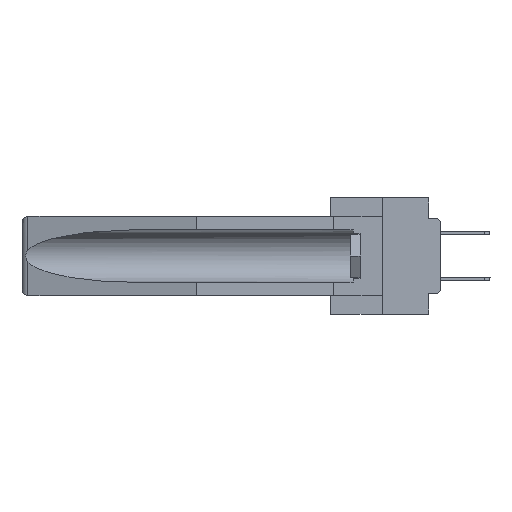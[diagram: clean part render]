
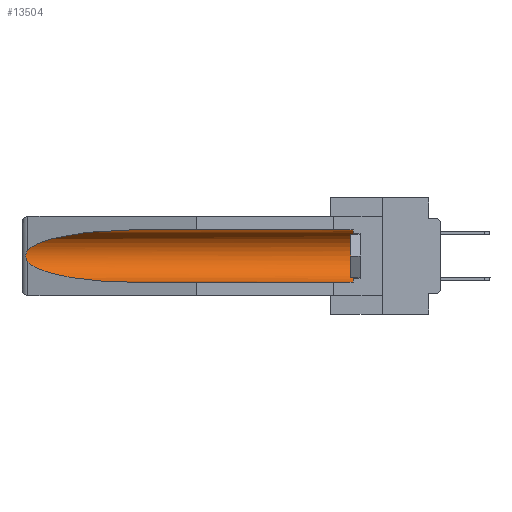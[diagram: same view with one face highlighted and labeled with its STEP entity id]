
A CAD part, left-side view. The second image highlights one B-rep face of the part: STEP entity #13504.
In plain terms, the highlighted cylindrical face has radius 2.857 mm (diameter 5.715 mm), a partial arc.
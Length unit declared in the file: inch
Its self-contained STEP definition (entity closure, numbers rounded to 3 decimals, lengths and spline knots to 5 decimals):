
#193 = ORIENTED_EDGE ( 'NONE', *, *, #30824, .T. ) ;
#629 = VERTEX_POINT ( 'NONE', #15330 ) ;
#697 = CARTESIAN_POINT ( 'NONE',  ( 0.2675, 1.53308, -0.17534 ) ) ;
#832 = CARTESIAN_POINT ( 'NONE',  ( 0.2673, 1.5327, -0.16383 ) ) ;
#1252 = DIRECTION ( 'NONE',  ( 0., 0., 1. ) ) ;
#2626 = VERTEX_POINT ( 'NONE', #10503 ) ;
#2793 = CARTESIAN_POINT ( 'NONE',  ( 0.25451, 1.48313, -0.24835 ) ) ;
#4478 = CARTESIAN_POINT ( 'NONE',  ( 0.155, 1.07973, -0.059 ) ) ;
#4939 = CARTESIAN_POINT ( 'NONE',  ( 0.26537, 1.52718, -0.14972 ) ) ;
#5345 = ORIENTED_EDGE ( 'NONE', *, *, #19482, .T. ) ;
#5574 = EDGE_CURVE ( 'NONE', #11075, #629, #6976, .T. ) ;
#6782 = CARTESIAN_POINT ( 'NONE',  ( 0.26537, 1.52718, -0.19328 ) ) ;
#6976 =( BOUNDED_CURVE ( )  B_SPLINE_CURVE ( 3, ( #32112, #2793, #9808, #11734 ),
 .UNSPECIFIED., .F., .F. ) 
 B_SPLINE_CURVE_WITH_KNOTS ( ( 4, 4 ),
 ( 0.1948, 1.5708 ),
 .UNSPECIFIED. ) 
 CURVE ( )  GEOMETRIC_REPRESENTATION_ITEM ( )  RATIONAL_B_SPLINE_CURVE ( ( 1., 0.848, 0.848, 1. ) ) 
 REPRESENTATION_ITEM ( '' )  );
#7570 = AXIS2_PLACEMENT_3D ( 'NONE', #27315, #30630, #1252 ) ;
#8059 = CARTESIAN_POINT ( 'NONE',  ( 0.155, 1.07973, -0.059 ) ) ;
#8089 = CYLINDRICAL_SURFACE ( 'NONE', #7570, 0.1125 ) ;
#8916 = ORIENTED_EDGE ( 'NONE', *, *, #30125, .F. ) ;
#9808 = CARTESIAN_POINT ( 'NONE',  ( 0.21114, 1.30732, -0.284 ) ) ;
#9833 = CARTESIAN_POINT ( 'NONE',  ( 0.26597, 1.52961, -0.15275 ) ) ;
#10503 = CARTESIAN_POINT ( 'NONE',  ( 0.155, 0.126, -0.059 ) ) ;
#11075 = VERTEX_POINT ( 'NONE', #17064 ) ;
#11184 = CARTESIAN_POINT ( 'NONE',  ( 0.155, -0.30754, -0.059 ) ) ;
#11734 = CARTESIAN_POINT ( 'NONE',  ( 0.155, 1.07973, -0.284 ) ) ;
#11751 = EDGE_CURVE ( 'NONE', #36220, #2626, #14532, .T. ) ;
#12154 = DIRECTION ( 'NONE',  ( 0., 1., 0. ) ) ;
#12228 = CARTESIAN_POINT ( 'NONE',  ( 0.2673, 1.53269, -0.17917 ) ) ;
#12787 = ORIENTED_EDGE ( 'NONE', *, *, #29955, .T. ) ;
#13504 = ADVANCED_FACE ( 'NONE', ( #25266 ), #8089, .F. ) ;
#13852 = CARTESIAN_POINT ( 'NONE',  ( 0.21114, 1.30732, -0.059 ) ) ;
#13968 = LINE ( 'NONE', #35691, #26182 ) ;
#14532 = CIRCLE ( 'NONE', #32804, 0.1125 ) ;
#15234 = CARTESIAN_POINT ( 'NONE',  ( 0.26654, 1.53092, -0.15636 ) ) ;
#15330 = CARTESIAN_POINT ( 'NONE',  ( 0.155, 1.07973, -0.284 ) ) ;
#15476 = CARTESIAN_POINT ( 'NONE',  ( 0.2675, 1.53308, -0.16763 ) ) ;
#15528 = ORIENTED_EDGE ( 'NONE', *, *, #11751, .T. ) ;
#15782 = B_SPLINE_CURVE_WITH_KNOTS ( 'NONE', 3,
 ( #21436, #9833, #15234, #832, #15476, #697, #12228, #20925, #29967, #6782 ),
 .UNSPECIFIED., .F., .F.,
 ( 4, 2, 2, 2, 4 ),
 ( 0., 0.00029, 0.00058, 0.00087, 0.00117 ),
 .UNSPECIFIED. ) ;
#16935 = DIRECTION ( 'NONE',  ( 0., 0., 1. ) ) ;
#16987 = CARTESIAN_POINT ( 'NONE',  ( 0.26537, 1.52718, -0.14972 ) ) ;
#17064 = CARTESIAN_POINT ( 'NONE',  ( 0.26537, 1.52718, -0.19328 ) ) ;
#17321 = DIRECTION ( 'NONE',  ( 0., -1., 0. ) ) ;
#19482 = EDGE_CURVE ( 'NONE', #35399, #32758, #20863, .T. ) ;
#19641 = CARTESIAN_POINT ( 'NONE',  ( 0.25451, 1.48313, -0.09465 ) ) ;
#20863 =( BOUNDED_CURVE ( )  B_SPLINE_CURVE ( 3, ( #8059, #13852, #19641, #16987 ),
 .UNSPECIFIED., .F., .F. ) 
 B_SPLINE_CURVE_WITH_KNOTS ( ( 4, 4 ),
 ( 4.71239, 6.08839 ),
 .UNSPECIFIED. ) 
 CURVE ( )  GEOMETRIC_REPRESENTATION_ITEM ( )  RATIONAL_B_SPLINE_CURVE ( ( 1., 0.848, 0.848, 1. ) ) 
 REPRESENTATION_ITEM ( '' )  );
#20925 = CARTESIAN_POINT ( 'NONE',  ( 0.26655, 1.53094, -0.18657 ) ) ;
#21436 = CARTESIAN_POINT ( 'NONE',  ( 0.26537, 1.52718, -0.14972 ) ) ;
#25266 = FACE_OUTER_BOUND ( 'NONE', #28109, .T. ) ;
#26182 = VECTOR ( 'NONE', #12154, 39.37008 ) ;
#27315 = CARTESIAN_POINT ( 'NONE',  ( 0.155, -0.30754, -0.1715 ) ) ;
#27554 = ORIENTED_EDGE ( 'NONE', *, *, #5574, .T. ) ;
#28109 = EDGE_LOOP ( 'NONE', ( #5345, #193, #27554, #8916, #15528, #12787 ) ) ;
#29359 = DIRECTION ( 'NONE',  ( 0., 1., 0. ) ) ;
#29955 = EDGE_CURVE ( 'NONE', #2626, #35399, #37103, .T. ) ;
#29967 = CARTESIAN_POINT ( 'NONE',  ( 0.26597, 1.5296, -0.19026 ) ) ;
#30125 = EDGE_CURVE ( 'NONE', #36220, #629, #13968, .T. ) ;
#30630 = DIRECTION ( 'NONE',  ( 0., 1., 0. ) ) ;
#30824 = EDGE_CURVE ( 'NONE', #32758, #11075, #15782, .T. ) ;
#31512 = CARTESIAN_POINT ( 'NONE',  ( 0.155, 0.126, -0.284 ) ) ;
#32112 = CARTESIAN_POINT ( 'NONE',  ( 0.26537, 1.52718, -0.19328 ) ) ;
#32758 = VERTEX_POINT ( 'NONE', #4939 ) ;
#32804 = AXIS2_PLACEMENT_3D ( 'NONE', #34697, #17321, #16935 ) ;
#33032 = VECTOR ( 'NONE', #29359, 39.37008 ) ;
#34697 = CARTESIAN_POINT ( 'NONE',  ( 0.155, 0.126, -0.1715 ) ) ;
#35399 = VERTEX_POINT ( 'NONE', #4478 ) ;
#35691 = CARTESIAN_POINT ( 'NONE',  ( 0.155, -0.30754, -0.284 ) ) ;
#36220 = VERTEX_POINT ( 'NONE', #31512 ) ;
#37103 = LINE ( 'NONE', #11184, #33032 ) ;
